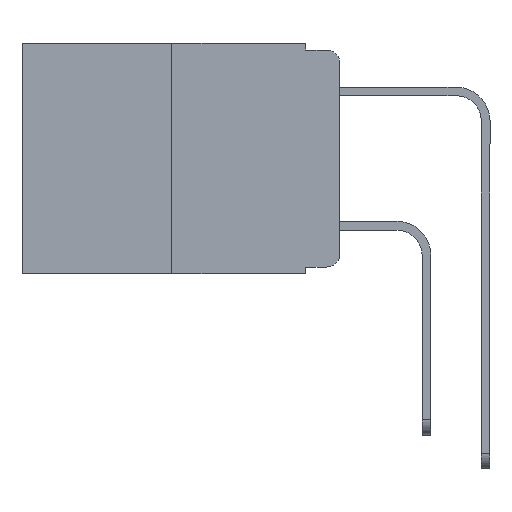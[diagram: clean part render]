
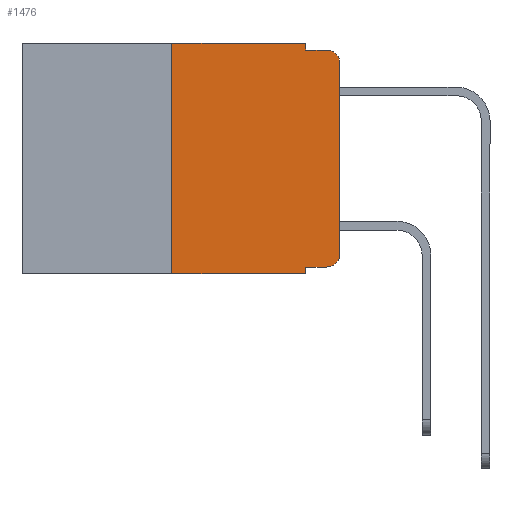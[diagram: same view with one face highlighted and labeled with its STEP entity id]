
A CAD part, left-side view. The second image highlights one B-rep face of the part: STEP entity #1476.
In plain terms, the highlighted planar face has unit normal (-1, 0, 0).
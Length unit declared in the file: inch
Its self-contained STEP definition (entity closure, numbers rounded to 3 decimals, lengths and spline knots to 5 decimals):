
#104 = AXIS2_PLACEMENT_3D ( 'NONE', #6399, #5156, #5366 ) ;
#263 = VERTEX_POINT ( 'NONE', #9066 ) ;
#293 = EDGE_CURVE ( 'NONE', #2348, #8115, #4080, .T. ) ;
#758 = CARTESIAN_POINT ( 'NONE',  ( 0., 0.25, 0. ) ) ;
#1003 = VECTOR ( 'NONE', #11396, 39.37008 ) ;
#1066 = CARTESIAN_POINT ( 'NONE',  ( 0., 0., 0. ) ) ;
#1079 = ORIENTED_EDGE ( 'NONE', *, *, #3420, .T. ) ;
#1158 = ORIENTED_EDGE ( 'NONE', *, *, #10434, .F. ) ;
#1244 = VECTOR ( 'NONE', #3588, 39.37008 ) ;
#1256 = FACE_OUTER_BOUND ( 'NONE', #3124, .T. ) ;
#1429 = ORIENTED_EDGE ( 'NONE', *, *, #5558, .T. ) ;
#1476 = ADVANCED_FACE ( 'NONE', ( #1256 ), #9742, .F. ) ;
#1714 = CARTESIAN_POINT ( 'NONE',  ( 0., 0., -0.03 ) ) ;
#1917 = CIRCLE ( 'NONE', #8912, 0.02 ) ;
#2010 = VECTOR ( 'NONE', #6082, 39.37008 ) ;
#2018 = DIRECTION ( 'NONE',  ( 0., 0., 1. ) ) ;
#2067 = DIRECTION ( 'NONE',  ( 0., -1., 0. ) ) ;
#2109 = CARTESIAN_POINT ( 'NONE',  ( 0., 0.051, -0.333 ) ) ;
#2157 = CARTESIAN_POINT ( 'NONE',  ( 0., 0.473, 0. ) ) ;
#2348 = VERTEX_POINT ( 'NONE', #7368 ) ;
#2498 = CARTESIAN_POINT ( 'NONE',  ( 0., 0.051, -0.343 ) ) ;
#2682 = CIRCLE ( 'NONE', #3552, 0.02 ) ;
#2961 = DIRECTION ( 'NONE',  ( -1., 0., 0. ) ) ;
#3124 = EDGE_LOOP ( 'NONE', ( #1079, #4911, #1158, #10967, #12182, #11571, #3927, #8017, #5609, #1429 ) ) ;
#3230 = LINE ( 'NONE', #2109, #9948 ) ;
#3420 = EDGE_CURVE ( 'NONE', #7890, #8887, #11955, .T. ) ;
#3552 = AXIS2_PLACEMENT_3D ( 'NONE', #5181, #11753, #6186 ) ;
#3588 = DIRECTION ( 'NONE',  ( 0., 0., -1. ) ) ;
#3593 = EDGE_CURVE ( 'NONE', #2348, #5473, #3230, .T. ) ;
#3618 = LINE ( 'NONE', #3818, #1003 ) ;
#3818 = CARTESIAN_POINT ( 'NONE',  ( 0., 0.25, 0. ) ) ;
#3912 = LINE ( 'NONE', #2157, #11173 ) ;
#3927 = ORIENTED_EDGE ( 'NONE', *, *, #10700, .T. ) ;
#4054 = VERTEX_POINT ( 'NONE', #5810 ) ;
#4080 = LINE ( 'NONE', #10539, #8847 ) ;
#4101 = CARTESIAN_POINT ( 'NONE',  ( 0., 0.02, -0.333 ) ) ;
#4721 = CARTESIAN_POINT ( 'NONE',  ( 0., 0.473, -0.343 ) ) ;
#4746 = VECTOR ( 'NONE', #2018, 39.37008 ) ;
#4911 = ORIENTED_EDGE ( 'NONE', *, *, #5376, .T. ) ;
#5156 = DIRECTION ( 'NONE',  ( 1., 0., 0. ) ) ;
#5181 = CARTESIAN_POINT ( 'NONE',  ( 0., 0.02, -0.313 ) ) ;
#5366 = DIRECTION ( 'NONE',  ( 0., 0., -1. ) ) ;
#5376 = EDGE_CURVE ( 'NONE', #8887, #4054, #1917, .T. ) ;
#5473 = VERTEX_POINT ( 'NONE', #4101 ) ;
#5558 = EDGE_CURVE ( 'NONE', #5473, #7890, #2682, .T. ) ;
#5563 = LINE ( 'NONE', #4721, #10272 ) ;
#5609 = ORIENTED_EDGE ( 'NONE', *, *, #3593, .T. ) ;
#5737 = DIRECTION ( 'NONE',  ( 0., -1., 0. ) ) ;
#5810 = CARTESIAN_POINT ( 'NONE',  ( 0., 0.02, -0.01 ) ) ;
#6082 = DIRECTION ( 'NONE',  ( 0., -1., 0. ) ) ;
#6103 = VERTEX_POINT ( 'NONE', #8838 ) ;
#6139 = DIRECTION ( 'NONE',  ( 0., -1., 0. ) ) ;
#6186 = DIRECTION ( 'NONE',  ( 0., 0., -1. ) ) ;
#6399 = CARTESIAN_POINT ( 'NONE',  ( 0., 0.473, 0. ) ) ;
#7368 = CARTESIAN_POINT ( 'NONE',  ( 0., 0.051, -0.333 ) ) ;
#7890 = VERTEX_POINT ( 'NONE', #8919 ) ;
#7963 = VERTEX_POINT ( 'NONE', #8041 ) ;
#8017 = ORIENTED_EDGE ( 'NONE', *, *, #293, .F. ) ;
#8041 = CARTESIAN_POINT ( 'NONE',  ( 0., 0.25, -0.343 ) ) ;
#8115 = VERTEX_POINT ( 'NONE', #2498 ) ;
#8155 = CARTESIAN_POINT ( 'NONE',  ( 0., 0.051, -0.01 ) ) ;
#8318 = EDGE_CURVE ( 'NONE', #7963, #8910, #3618, .T. ) ;
#8731 = CARTESIAN_POINT ( 'NONE',  ( 0., 0.02, -0.03 ) ) ;
#8733 = DIRECTION ( 'NONE',  ( 0., 0., -1. ) ) ;
#8838 = CARTESIAN_POINT ( 'NONE',  ( 0., 0.051, -0.01 ) ) ;
#8847 = VECTOR ( 'NONE', #8733, 39.37008 ) ;
#8887 = VERTEX_POINT ( 'NONE', #1714 ) ;
#8910 = VERTEX_POINT ( 'NONE', #758 ) ;
#8912 = AXIS2_PLACEMENT_3D ( 'NONE', #8731, #2961, #9669 ) ;
#8919 = CARTESIAN_POINT ( 'NONE',  ( 0., 0., -0.313 ) ) ;
#9066 = CARTESIAN_POINT ( 'NONE',  ( 0., 0.051, 0. ) ) ;
#9255 = LINE ( 'NONE', #10238, #1244 ) ;
#9417 = LINE ( 'NONE', #8155, #2010 ) ;
#9669 = DIRECTION ( 'NONE',  ( 0., 0., -1. ) ) ;
#9742 = PLANE ( 'NONE',  #104 ) ;
#9822 = EDGE_CURVE ( 'NONE', #8910, #263, #3912, .T. ) ;
#9948 = VECTOR ( 'NONE', #2067, 39.37008 ) ;
#10238 = CARTESIAN_POINT ( 'NONE',  ( 0., 0.051, 0. ) ) ;
#10272 = VECTOR ( 'NONE', #5737, 39.37008 ) ;
#10434 = EDGE_CURVE ( 'NONE', #6103, #4054, #9417, .T. ) ;
#10539 = CARTESIAN_POINT ( 'NONE',  ( 0., 0.051, 0. ) ) ;
#10700 = EDGE_CURVE ( 'NONE', #7963, #8115, #5563, .T. ) ;
#10967 = ORIENTED_EDGE ( 'NONE', *, *, #11067, .F. ) ;
#11067 = EDGE_CURVE ( 'NONE', #263, #6103, #9255, .T. ) ;
#11173 = VECTOR ( 'NONE', #6139, 39.37008 ) ;
#11396 = DIRECTION ( 'NONE',  ( 0., 0., 1. ) ) ;
#11571 = ORIENTED_EDGE ( 'NONE', *, *, #8318, .F. ) ;
#11753 = DIRECTION ( 'NONE',  ( -1., 0., 0. ) ) ;
#11955 = LINE ( 'NONE', #1066, #4746 ) ;
#12182 = ORIENTED_EDGE ( 'NONE', *, *, #9822, .F. ) ;
